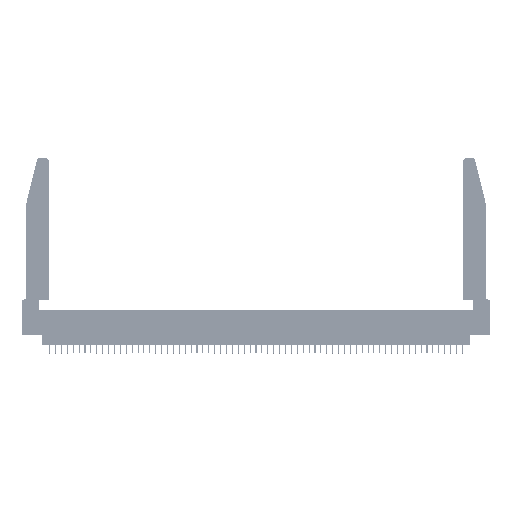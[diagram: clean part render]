
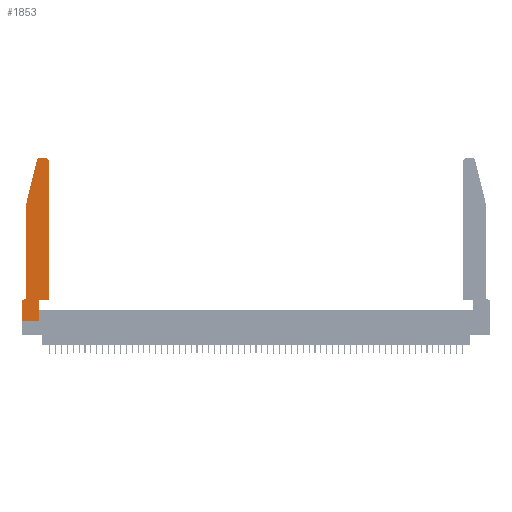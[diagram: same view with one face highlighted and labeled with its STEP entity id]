
A CAD part, top view. The second image highlights one B-rep face of the part: STEP entity #1853.
In plain terms, the highlighted planar face has unit normal (0, 0, 1).
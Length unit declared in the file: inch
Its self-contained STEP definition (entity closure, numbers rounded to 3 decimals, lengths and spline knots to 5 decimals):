
#27 = LINE ( 'NONE', #30755, #18030 ) ;
#43 = VECTOR ( 'NONE', #5443, 39.37008 ) ;
#293 = CARTESIAN_POINT ( 'NONE',  ( 0.4505, 0.35, 0.37 ) ) ;
#651 = VERTEX_POINT ( 'NONE', #53872 ) ;
#692 = DIRECTION ( 'NONE',  ( -1., 0., 0. ) ) ;
#832 = DIRECTION ( 'NONE',  ( 0., 0., -1. ) ) ;
#1267 = ORIENTED_EDGE ( 'NONE', *, *, #9916, .T. ) ;
#1648 = CARTESIAN_POINT ( 'NONE',  ( 0.2865, 0.35, 0.37 ) ) ;
#1796 = CARTESIAN_POINT ( 'NONE',  ( 0., 0.35, 0.37 ) ) ;
#1853 = ADVANCED_FACE ( 'NONE', ( #37159 ), #41193, .T. ) ;
#2940 = EDGE_CURVE ( 'NONE', #42988, #4768, #42574, .T. ) ;
#3457 = DIRECTION ( 'NONE',  ( 1., 0., 0. ) ) ;
#4768 = VERTEX_POINT ( 'NONE', #30398 ) ;
#4881 = EDGE_CURVE ( 'NONE', #6325, #42988, #55639, .T. ) ;
#5443 = DIRECTION ( 'NONE',  ( 0., 1., 0. ) ) ;
#5487 = CARTESIAN_POINT ( 'NONE',  ( 0.2865, 0., 0.37 ) ) ;
#6035 = AXIS2_PLACEMENT_3D ( 'NONE', #40513, #832, #10287 ) ;
#6055 = VECTOR ( 'NONE', #3457, 39.37008 ) ;
#6325 = VERTEX_POINT ( 'NONE', #5487 ) ;
#7180 = VECTOR ( 'NONE', #37219, 39.37008 ) ;
#7225 = EDGE_CURVE ( 'NONE', #32717, #49231, #50970, .T. ) ;
#7483 = CARTESIAN_POINT ( 'NONE',  ( 0., 0., 0.37 ) ) ;
#7600 = AXIS2_PLACEMENT_3D ( 'NONE', #18450, #36078, #49828 ) ;
#8759 = CARTESIAN_POINT ( 'NONE',  ( 0., 0., 0.37 ) ) ;
#9168 = EDGE_CURVE ( 'NONE', #35447, #32717, #19698, .T. ) ;
#9916 = EDGE_CURVE ( 'NONE', #18380, #35447, #31684, .T. ) ;
#10128 = DIRECTION ( 'NONE',  ( 0., 0., 1. ) ) ;
#10287 = DIRECTION ( 'NONE',  ( -1., 0., 0. ) ) ;
#10408 = CARTESIAN_POINT ( 'NONE',  ( 0.4205, 2.75, 0.37 ) ) ;
#10678 = CARTESIAN_POINT ( 'NONE',  ( 0.0755, 2., 0.37 ) ) ;
#11263 = CARTESIAN_POINT ( 'NONE',  ( 0.284, 2.75, 0.37 ) ) ;
#12012 = LINE ( 'NONE', #38500, #45982 ) ;
#14434 = LINE ( 'NONE', #49254, #22581 ) ;
#16042 = DIRECTION ( 'NONE',  ( 0., 0., 1. ) ) ;
#16215 = CARTESIAN_POINT ( 'NONE',  ( 0.0055, 0.35, 0.37 ) ) ;
#16899 = CARTESIAN_POINT ( 'NONE',  ( 0.0755, 0.35, 0.37 ) ) ;
#18030 = VECTOR ( 'NONE', #48047, 39.37008 ) ;
#18380 = VERTEX_POINT ( 'NONE', #26088 ) ;
#18450 = CARTESIAN_POINT ( 'NONE',  ( 0.284, 2.72, 0.37 ) ) ;
#19282 = ORIENTED_EDGE ( 'NONE', *, *, #30419, .T. ) ;
#19698 = CIRCLE ( 'NONE', #6035, 0.07 ) ;
#19711 = VERTEX_POINT ( 'NONE', #48561 ) ;
#20046 = DIRECTION ( 'NONE',  ( 1., 0., 0. ) ) ;
#20743 = CARTESIAN_POINT ( 'NONE',  ( 0.2865, 0.35, 0.37 ) ) ;
#21312 = CIRCLE ( 'NONE', #7600, 0.03 ) ;
#21393 = CARTESIAN_POINT ( 'NONE',  ( 0., 0.35, 0.37 ) ) ;
#21637 = ORIENTED_EDGE ( 'NONE', *, *, #30465, .T. ) ;
#22581 = VECTOR ( 'NONE', #692, 39.37008 ) ;
#22690 = ORIENTED_EDGE ( 'NONE', *, *, #7225, .T. ) ;
#22849 = ORIENTED_EDGE ( 'NONE', *, *, #37325, .T. ) ;
#23228 = VERTEX_POINT ( 'NONE', #11263 ) ;
#24549 = EDGE_CURVE ( 'NONE', #23228, #651, #21312, .T. ) ;
#25758 = ORIENTED_EDGE ( 'NONE', *, *, #37598, .T. ) ;
#26088 = CARTESIAN_POINT ( 'NONE',  ( 0.0755, 2., 0.37 ) ) ;
#27914 = ORIENTED_EDGE ( 'NONE', *, *, #9168, .T. ) ;
#29785 = VERTEX_POINT ( 'NONE', #10408 ) ;
#30398 = CARTESIAN_POINT ( 'NONE',  ( 0.4505, 0.35, 0.37 ) ) ;
#30419 = EDGE_CURVE ( 'NONE', #19711, #29785, #33601, .T. ) ;
#30465 = EDGE_CURVE ( 'NONE', #34978, #6325, #46862, .T. ) ;
#30755 = CARTESIAN_POINT ( 'NONE',  ( 0., 0., 0.37 ) ) ;
#31656 = ORIENTED_EDGE ( 'NONE', *, *, #47248, .T. ) ;
#31684 = LINE ( 'NONE', #10678, #43447 ) ;
#32717 = VERTEX_POINT ( 'NONE', #16215 ) ;
#33601 = CIRCLE ( 'NONE', #47387, 0.03 ) ;
#34978 = VERTEX_POINT ( 'NONE', #8759 ) ;
#35256 = ORIENTED_EDGE ( 'NONE', *, *, #2940, .T. ) ;
#35447 = VERTEX_POINT ( 'NONE', #56160 ) ;
#35671 = LINE ( 'NONE', #293, #43 ) ;
#36078 = DIRECTION ( 'NONE',  ( 0., 0., 1. ) ) ;
#37138 = DIRECTION ( 'NONE',  ( 0., -1., 0. ) ) ;
#37159 = FACE_OUTER_BOUND ( 'NONE', #52487, .T. ) ;
#37219 = DIRECTION ( 'NONE',  ( 0., 1., 0. ) ) ;
#37325 = EDGE_CURVE ( 'NONE', #4768, #19711, #35671, .T. ) ;
#37598 = EDGE_CURVE ( 'NONE', #651, #18380, #12012, .T. ) ;
#38253 = CARTESIAN_POINT ( 'NONE',  ( 0.4505, 0.35, 0.37 ) ) ;
#38500 = CARTESIAN_POINT ( 'NONE',  ( 0.0755, 2., 0.37 ) ) ;
#40513 = CARTESIAN_POINT ( 'NONE',  ( 0.0055, 0.42, 0.37 ) ) ;
#41193 = PLANE ( 'NONE',  #43853 ) ;
#42574 = LINE ( 'NONE', #38253, #45754 ) ;
#42988 = VERTEX_POINT ( 'NONE', #1648 ) ;
#43447 = VECTOR ( 'NONE', #37138, 39.37008 ) ;
#43853 = AXIS2_PLACEMENT_3D ( 'NONE', #1796, #10128, #54719 ) ;
#45728 = ORIENTED_EDGE ( 'NONE', *, *, #24549, .T. ) ;
#45754 = VECTOR ( 'NONE', #51792, 39.37008 ) ;
#45982 = VECTOR ( 'NONE', #56040, 39.37008 ) ;
#46351 = EDGE_CURVE ( 'NONE', #29785, #23228, #14434, .T. ) ;
#46862 = LINE ( 'NONE', #7483, #6055 ) ;
#47248 = EDGE_CURVE ( 'NONE', #49231, #34978, #27, .T. ) ;
#47387 = AXIS2_PLACEMENT_3D ( 'NONE', #56083, #16042, #20046 ) ;
#48008 = DIRECTION ( 'NONE',  ( -1., 0., 0. ) ) ;
#48047 = DIRECTION ( 'NONE',  ( 0., -1., 0. ) ) ;
#48561 = CARTESIAN_POINT ( 'NONE',  ( 0.4505, 2.72, 0.37 ) ) ;
#49027 = VECTOR ( 'NONE', #48008, 39.37008 ) ;
#49231 = VERTEX_POINT ( 'NONE', #21393 ) ;
#49254 = CARTESIAN_POINT ( 'NONE',  ( 0.2605, 2.75, 0.37 ) ) ;
#49828 = DIRECTION ( 'NONE',  ( 1., 0., 0. ) ) ;
#50970 = LINE ( 'NONE', #16899, #49027 ) ;
#51792 = DIRECTION ( 'NONE',  ( 1., 0., 0. ) ) ;
#52487 = EDGE_LOOP ( 'NONE', ( #55640, #45728, #25758, #1267, #27914, #22690, #31656, #21637, #53096, #35256, #22849, #19282 ) ) ;
#53096 = ORIENTED_EDGE ( 'NONE', *, *, #4881, .T. ) ;
#53872 = CARTESIAN_POINT ( 'NONE',  ( 0.25487, 2.72718, 0.37 ) ) ;
#54719 = DIRECTION ( 'NONE',  ( 1., 0., 0. ) ) ;
#55639 = LINE ( 'NONE', #20743, #7180 ) ;
#55640 = ORIENTED_EDGE ( 'NONE', *, *, #46351, .T. ) ;
#56040 = DIRECTION ( 'NONE',  ( -0.239, -0.971, 0. ) ) ;
#56083 = CARTESIAN_POINT ( 'NONE',  ( 0.4205, 2.72, 0.37 ) ) ;
#56160 = CARTESIAN_POINT ( 'NONE',  ( 0.0755, 0.42, 0.37 ) ) ;
